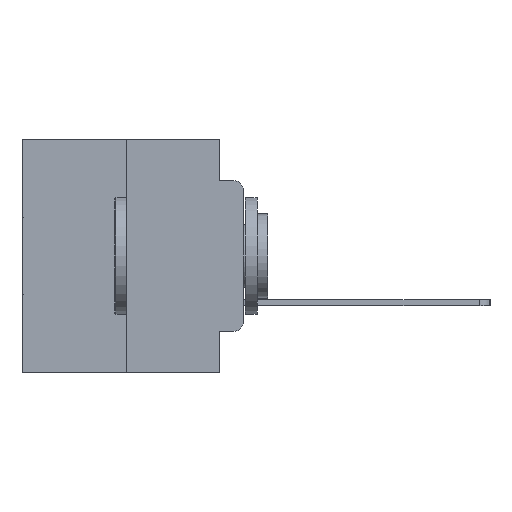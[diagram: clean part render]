
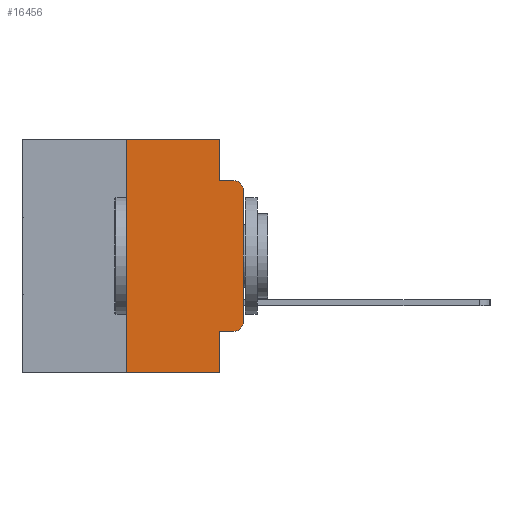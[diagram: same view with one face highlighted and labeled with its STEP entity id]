
A CAD part, left-side view. The second image highlights one B-rep face of the part: STEP entity #16456.
In plain terms, the highlighted planar face has unit normal (-1, 0, 0).
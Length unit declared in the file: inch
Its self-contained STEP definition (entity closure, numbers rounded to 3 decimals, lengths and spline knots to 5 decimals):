
#288 = VECTOR ( 'NONE', #18714, 39.37008 ) ;
#419 = ORIENTED_EDGE ( 'NONE', *, *, #503, .T. ) ;
#502 = CARTESIAN_POINT ( 'NONE',  ( 0., 0.051, 0. ) ) ;
#503 = EDGE_CURVE ( 'NONE', #9029, #17961, #5859, .T. ) ;
#555 = CARTESIAN_POINT ( 'NONE',  ( 0., 0.25, 0. ) ) ;
#744 = EDGE_CURVE ( 'NONE', #3703, #9990, #14148, .T. ) ;
#745 = CARTESIAN_POINT ( 'NONE',  ( 0., 0.051, -0.4115 ) ) ;
#815 = EDGE_LOOP ( 'NONE', ( #28869, #24278, #15524, #10113, #22478, #23196, #17707, #12273, #419, #2750 ) ) ;
#1056 = DIRECTION ( 'NONE',  ( 0., 0., -1. ) ) ;
#1120 = LINE ( 'NONE', #24525, #12904 ) ;
#1138 = VERTEX_POINT ( 'NONE', #10575 ) ;
#1546 = CARTESIAN_POINT ( 'NONE',  ( 0., 0.051, -0.5 ) ) ;
#1769 = VERTEX_POINT ( 'NONE', #24590 ) ;
#2072 = CARTESIAN_POINT ( 'NONE',  ( 0., 0.051, 0. ) ) ;
#2102 = VECTOR ( 'NONE', #16175, 39.37008 ) ;
#2750 = ORIENTED_EDGE ( 'NONE', *, *, #29215, .T. ) ;
#3581 = VECTOR ( 'NONE', #8614, 39.37008 ) ;
#3703 = VERTEX_POINT ( 'NONE', #555 ) ;
#3808 = EDGE_CURVE ( 'NONE', #9029, #23172, #25738, .T. ) ;
#3882 = CARTESIAN_POINT ( 'NONE',  ( 0., 0.051, -0.0885 ) ) ;
#4020 = PLANE ( 'NONE',  #25130 ) ;
#4178 = VERTEX_POINT ( 'NONE', #12507 ) ;
#4269 = CARTESIAN_POINT ( 'NONE',  ( 0., 0.02, -0.3915 ) ) ;
#5386 = EDGE_CURVE ( 'NONE', #4178, #3703, #1120, .T. ) ;
#5804 = EDGE_CURVE ( 'NONE', #4178, #23172, #19061, .T. ) ;
#5859 = LINE ( 'NONE', #25794, #2102 ) ;
#6412 = DIRECTION ( 'NONE',  ( 1., 0., 0. ) ) ;
#6642 = DIRECTION ( 'NONE',  ( 0., 0., -1. ) ) ;
#6952 = EDGE_CURVE ( 'NONE', #9990, #25956, #30096, .T. ) ;
#6984 = LINE ( 'NONE', #18495, #18597 ) ;
#8271 = DIRECTION ( 'NONE',  ( 0., 0., 1. ) ) ;
#8536 = EDGE_CURVE ( 'NONE', #25956, #1138, #28256, .T. ) ;
#8614 = DIRECTION ( 'NONE',  ( 0., -1., 0. ) ) ;
#9029 = VERTEX_POINT ( 'NONE', #745 ) ;
#9834 = AXIS2_PLACEMENT_3D ( 'NONE', #4269, #20535, #6642 ) ;
#9990 = VERTEX_POINT ( 'NONE', #502 ) ;
#10094 = EDGE_CURVE ( 'NONE', #1769, #1138, #19810, .T. ) ;
#10113 = ORIENTED_EDGE ( 'NONE', *, *, #6952, .F. ) ;
#10575 = CARTESIAN_POINT ( 'NONE',  ( 0., 0.02, -0.0885 ) ) ;
#11622 = EDGE_CURVE ( 'NONE', #15360, #1769, #6984, .T. ) ;
#11717 = VECTOR ( 'NONE', #29861, 39.37008 ) ;
#12273 = ORIENTED_EDGE ( 'NONE', *, *, #3808, .F. ) ;
#12507 = CARTESIAN_POINT ( 'NONE',  ( 0., 0.25, -0.5 ) ) ;
#12904 = VECTOR ( 'NONE', #8271, 39.37008 ) ;
#13980 = DIRECTION ( 'NONE',  ( 0., -1., 0. ) ) ;
#14148 = LINE ( 'NONE', #21601, #26541 ) ;
#15111 = DIRECTION ( 'NONE',  ( -1., 0., 0. ) ) ;
#15360 = VERTEX_POINT ( 'NONE', #18625 ) ;
#15524 = ORIENTED_EDGE ( 'NONE', *, *, #8536, .F. ) ;
#15926 = CARTESIAN_POINT ( 'NONE',  ( 0., 0.051, 0. ) ) ;
#16175 = DIRECTION ( 'NONE',  ( 0., -1., 0. ) ) ;
#16456 = ADVANCED_FACE ( 'NONE', ( #17980 ), #4020, .F. ) ;
#17284 = CIRCLE ( 'NONE', #9834, 0.02 ) ;
#17707 = ORIENTED_EDGE ( 'NONE', *, *, #5804, .T. ) ;
#17961 = VERTEX_POINT ( 'NONE', #20417 ) ;
#17980 = FACE_OUTER_BOUND ( 'NONE', #815, .T. ) ;
#18275 = DIRECTION ( 'NONE',  ( 0., 0., -1. ) ) ;
#18495 = CARTESIAN_POINT ( 'NONE',  ( 0., 0., 0. ) ) ;
#18597 = VECTOR ( 'NONE', #20818, 39.37008 ) ;
#18625 = CARTESIAN_POINT ( 'NONE',  ( 0., 0., -0.3915 ) ) ;
#18714 = DIRECTION ( 'NONE',  ( 0., -1., 0. ) ) ;
#18730 = AXIS2_PLACEMENT_3D ( 'NONE', #28946, #15111, #1056 ) ;
#18924 = CARTESIAN_POINT ( 'NONE',  ( 0., 0.051, -0.0885 ) ) ;
#19061 = LINE ( 'NONE', #21044, #288 ) ;
#19561 = VECTOR ( 'NONE', #18275, 39.37008 ) ;
#19810 = CIRCLE ( 'NONE', #18730, 0.02 ) ;
#20417 = CARTESIAN_POINT ( 'NONE',  ( 0., 0.02, -0.4115 ) ) ;
#20535 = DIRECTION ( 'NONE',  ( -1., 0., 0. ) ) ;
#20818 = DIRECTION ( 'NONE',  ( 0., 0., 1. ) ) ;
#21044 = CARTESIAN_POINT ( 'NONE',  ( 0., 0.473, -0.5 ) ) ;
#21601 = CARTESIAN_POINT ( 'NONE',  ( 0., 0.473, 0. ) ) ;
#22478 = ORIENTED_EDGE ( 'NONE', *, *, #744, .F. ) ;
#22667 = DIRECTION ( 'NONE',  ( 0., 0., -1. ) ) ;
#23172 = VERTEX_POINT ( 'NONE', #1546 ) ;
#23196 = ORIENTED_EDGE ( 'NONE', *, *, #5386, .F. ) ;
#24278 = ORIENTED_EDGE ( 'NONE', *, *, #10094, .T. ) ;
#24525 = CARTESIAN_POINT ( 'NONE',  ( 0., 0.25, 0. ) ) ;
#24590 = CARTESIAN_POINT ( 'NONE',  ( 0., 0., -0.1085 ) ) ;
#25130 = AXIS2_PLACEMENT_3D ( 'NONE', #29430, #6412, #22667 ) ;
#25738 = LINE ( 'NONE', #15926, #19561 ) ;
#25794 = CARTESIAN_POINT ( 'NONE',  ( 0., 0.051, -0.4115 ) ) ;
#25956 = VERTEX_POINT ( 'NONE', #18924 ) ;
#26541 = VECTOR ( 'NONE', #13980, 39.37008 ) ;
#28256 = LINE ( 'NONE', #3882, #3581 ) ;
#28869 = ORIENTED_EDGE ( 'NONE', *, *, #11622, .T. ) ;
#28946 = CARTESIAN_POINT ( 'NONE',  ( 0., 0.02, -0.1085 ) ) ;
#29215 = EDGE_CURVE ( 'NONE', #17961, #15360, #17284, .T. ) ;
#29430 = CARTESIAN_POINT ( 'NONE',  ( 0., 0.473, 0. ) ) ;
#29861 = DIRECTION ( 'NONE',  ( 0., 0., -1. ) ) ;
#30096 = LINE ( 'NONE', #2072, #11717 ) ;
